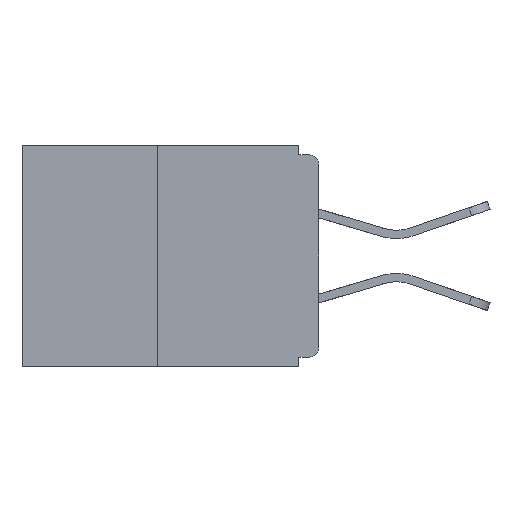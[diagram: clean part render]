
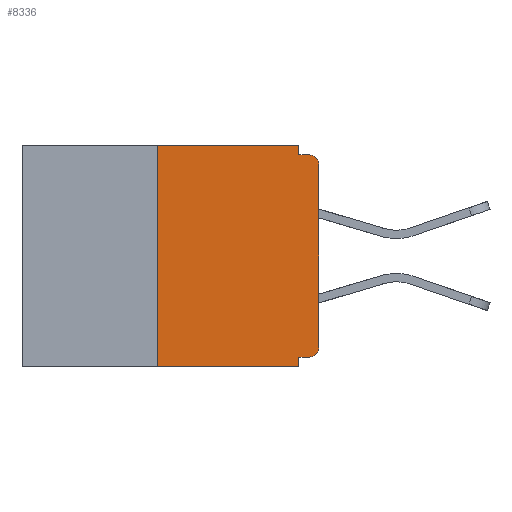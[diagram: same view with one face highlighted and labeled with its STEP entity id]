
A CAD part, left-side view. The second image highlights one B-rep face of the part: STEP entity #8336.
In plain terms, the highlighted planar face has unit normal (-1, 0, 0).
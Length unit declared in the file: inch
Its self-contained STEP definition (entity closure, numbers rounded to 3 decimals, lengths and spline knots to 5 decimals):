
#580 = VECTOR ( 'NONE', #5394, 39.37008 ) ;
#681 = CARTESIAN_POINT ( 'NONE',  ( 0., 0.25, 0. ) ) ;
#939 = LINE ( 'NONE', #18734, #580 ) ;
#975 = EDGE_CURVE ( 'NONE', #15162, #18680, #24957, .T. ) ;
#1282 = CARTESIAN_POINT ( 'NONE',  ( 0., 0.015, -0.328 ) ) ;
#1332 = AXIS2_PLACEMENT_3D ( 'NONE', #15004, #15095, #19490 ) ;
#2051 = AXIS2_PLACEMENT_3D ( 'NONE', #15514, #2473, #4617 ) ;
#2214 = DIRECTION ( 'NONE',  ( 0., -1., 0. ) ) ;
#2254 = VERTEX_POINT ( 'NONE', #1282 ) ;
#2473 = DIRECTION ( 'NONE',  ( -1., 0., 0. ) ) ;
#2905 = CARTESIAN_POINT ( 'NONE',  ( 0., 0.25, -0.343 ) ) ;
#3418 = DIRECTION ( 'NONE',  ( 0., 0., -1. ) ) ;
#3430 = VECTOR ( 'NONE', #25847, 39.37008 ) ;
#3522 = VERTEX_POINT ( 'NONE', #19675 ) ;
#3706 = VERTEX_POINT ( 'NONE', #18691 ) ;
#4180 = VECTOR ( 'NONE', #12491, 39.37008 ) ;
#4617 = DIRECTION ( 'NONE',  ( 0., 0., -1. ) ) ;
#4703 = ORIENTED_EDGE ( 'NONE', *, *, #26190, .T. ) ;
#4884 = VERTEX_POINT ( 'NONE', #25836 ) ;
#5278 = EDGE_LOOP ( 'NONE', ( #24157, #28157, #17324, #16700, #9204, #15981, #24570, #4703, #24129, #27368 ) ) ;
#5394 = DIRECTION ( 'NONE',  ( 0., 1., 0. ) ) ;
#5663 = LINE ( 'NONE', #16544, #27174 ) ;
#6052 = DIRECTION ( 'NONE',  ( 0., 0., 1. ) ) ;
#6480 = LINE ( 'NONE', #19265, #3430 ) ;
#6718 = CARTESIAN_POINT ( 'NONE',  ( 0., 0., -0.015 ) ) ;
#7444 = CARTESIAN_POINT ( 'NONE',  ( 0., 0., -0.03 ) ) ;
#7923 = AXIS2_PLACEMENT_3D ( 'NONE', #21078, #8070, #3418 ) ;
#8070 = DIRECTION ( 'NONE',  ( 1., 0., 0. ) ) ;
#8336 = ADVANCED_FACE ( 'NONE', ( #15090 ), #18853, .F. ) ;
#9204 = ORIENTED_EDGE ( 'NONE', *, *, #13138, .F. ) ;
#11716 = LINE ( 'NONE', #16968, #4180 ) ;
#12396 = VECTOR ( 'NONE', #24004, 39.37008 ) ;
#12491 = DIRECTION ( 'NONE',  ( 0., -1., 0. ) ) ;
#13138 = EDGE_CURVE ( 'NONE', #2254, #23743, #939, .T. ) ;
#13267 = EDGE_CURVE ( 'NONE', #20069, #26501, #5663, .T. ) ;
#14283 = VERTEX_POINT ( 'NONE', #16764 ) ;
#14877 = EDGE_CURVE ( 'NONE', #2254, #20069, #24672, .T. ) ;
#15004 = CARTESIAN_POINT ( 'NONE',  ( 0., 0.015, -0.313 ) ) ;
#15090 = FACE_OUTER_BOUND ( 'NONE', #5278, .T. ) ;
#15095 = DIRECTION ( 'NONE',  ( -1., 0., 0. ) ) ;
#15159 = CARTESIAN_POINT ( 'NONE',  ( 0., 0.25, 0. ) ) ;
#15162 = VERTEX_POINT ( 'NONE', #2905 ) ;
#15514 = CARTESIAN_POINT ( 'NONE',  ( 0., 0.015, -0.03 ) ) ;
#15981 = ORIENTED_EDGE ( 'NONE', *, *, #14877, .T. ) ;
#16049 = DIRECTION ( 'NONE',  ( 0., 0., -1. ) ) ;
#16544 = CARTESIAN_POINT ( 'NONE',  ( 0., 0., 0. ) ) ;
#16700 = ORIENTED_EDGE ( 'NONE', *, *, #21958, .F. ) ;
#16764 = CARTESIAN_POINT ( 'NONE',  ( 0., 0.031, -0.343 ) ) ;
#16968 = CARTESIAN_POINT ( 'NONE',  ( 0., 0.46, -0.343 ) ) ;
#17324 = ORIENTED_EDGE ( 'NONE', *, *, #27043, .T. ) ;
#17565 = VECTOR ( 'NONE', #2214, 39.37008 ) ;
#18258 = LINE ( 'NONE', #26496, #17565 ) ;
#18680 = VERTEX_POINT ( 'NONE', #15159 ) ;
#18691 = CARTESIAN_POINT ( 'NONE',  ( 0., 0.015, -0.015 ) ) ;
#18734 = CARTESIAN_POINT ( 'NONE',  ( 0., 0., -0.328 ) ) ;
#18834 = DIRECTION ( 'NONE',  ( 0., 0., 1. ) ) ;
#18853 = PLANE ( 'NONE',  #7923 ) ;
#19265 = CARTESIAN_POINT ( 'NONE',  ( 0., 0.031, -0.343 ) ) ;
#19490 = DIRECTION ( 'NONE',  ( 0., 0., -1. ) ) ;
#19675 = CARTESIAN_POINT ( 'NONE',  ( 0., 0.031, 0. ) ) ;
#20069 = VERTEX_POINT ( 'NONE', #26890 ) ;
#20465 = EDGE_CURVE ( 'NONE', #4884, #3706, #24005, .T. ) ;
#21078 = CARTESIAN_POINT ( 'NONE',  ( 0., 0.46, 0. ) ) ;
#21431 = CARTESIAN_POINT ( 'NONE',  ( 0., 0.031, -0.328 ) ) ;
#21681 = CIRCLE ( 'NONE', #2051, 0.015 ) ;
#21958 = EDGE_CURVE ( 'NONE', #23743, #14283, #6480, .T. ) ;
#23322 = EDGE_CURVE ( 'NONE', #3522, #4884, #28255, .T. ) ;
#23743 = VERTEX_POINT ( 'NONE', #21431 ) ;
#24004 = DIRECTION ( 'NONE',  ( 0., -1., 0. ) ) ;
#24005 = LINE ( 'NONE', #6718, #12396 ) ;
#24129 = ORIENTED_EDGE ( 'NONE', *, *, #20465, .F. ) ;
#24157 = ORIENTED_EDGE ( 'NONE', *, *, #25857, .F. ) ;
#24442 = CARTESIAN_POINT ( 'NONE',  ( 0., 0.031, 0. ) ) ;
#24486 = VECTOR ( 'NONE', #16049, 39.37008 ) ;
#24570 = ORIENTED_EDGE ( 'NONE', *, *, #13267, .T. ) ;
#24672 = CIRCLE ( 'NONE', #1332, 0.015 ) ;
#24957 = LINE ( 'NONE', #681, #25651 ) ;
#25651 = VECTOR ( 'NONE', #18834, 39.37008 ) ;
#25836 = CARTESIAN_POINT ( 'NONE',  ( 0., 0.031, -0.015 ) ) ;
#25847 = DIRECTION ( 'NONE',  ( 0., 0., -1. ) ) ;
#25857 = EDGE_CURVE ( 'NONE', #18680, #3522, #18258, .T. ) ;
#26190 = EDGE_CURVE ( 'NONE', #26501, #3706, #21681, .T. ) ;
#26496 = CARTESIAN_POINT ( 'NONE',  ( 0., 0.46, 0. ) ) ;
#26501 = VERTEX_POINT ( 'NONE', #7444 ) ;
#26890 = CARTESIAN_POINT ( 'NONE',  ( 0., 0., -0.313 ) ) ;
#27043 = EDGE_CURVE ( 'NONE', #15162, #14283, #11716, .T. ) ;
#27174 = VECTOR ( 'NONE', #6052, 39.37008 ) ;
#27368 = ORIENTED_EDGE ( 'NONE', *, *, #23322, .F. ) ;
#28157 = ORIENTED_EDGE ( 'NONE', *, *, #975, .F. ) ;
#28255 = LINE ( 'NONE', #24442, #24486 ) ;
